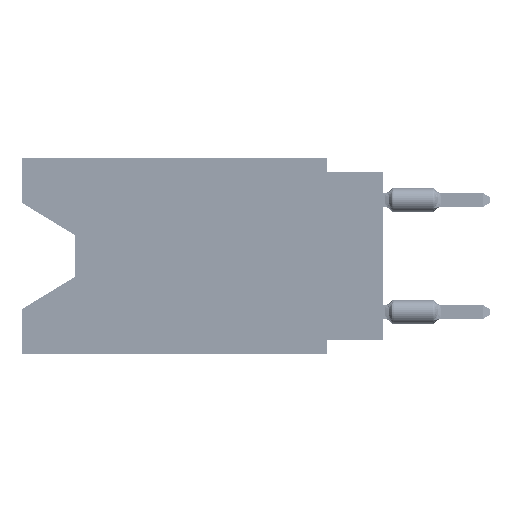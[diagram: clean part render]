
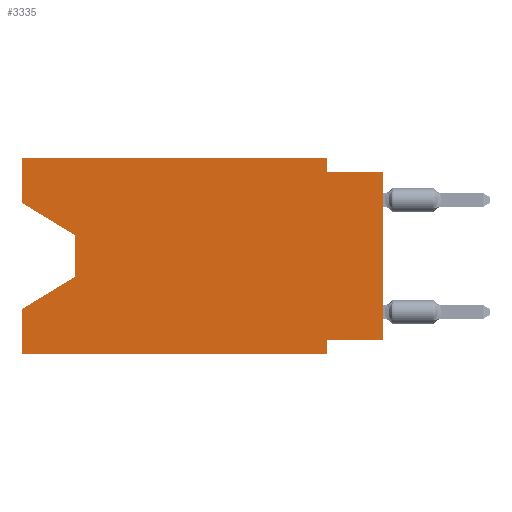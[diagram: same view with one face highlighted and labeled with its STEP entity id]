
A CAD part, left-side view. The second image highlights one B-rep face of the part: STEP entity #3335.
In plain terms, the highlighted planar face has unit normal (-1, 0, 0).
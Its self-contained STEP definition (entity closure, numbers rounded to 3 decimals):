
#1434 = VECTOR ( 'NONE', #78253, 1000. ) ;
#2372 = DIRECTION ( 'NONE',  ( 0., 0., 1. ) ) ;
#2408 = CARTESIAN_POINT ( 'NONE',  ( 0., 2.54, -8.89 ) ) ;
#3335 = ADVANCED_FACE ( 'NONE', ( #8210 ), #54023, .F. ) ;
#4043 = CARTESIAN_POINT ( 'NONE',  ( 0., 2.54, -8.255 ) ) ;
#4222 = CARTESIAN_POINT ( 'NONE',  ( 0., 13.97, -3.505 ) ) ;
#4319 = ORIENTED_EDGE ( 'NONE', *, *, #28063, .T. ) ;
#4534 = CARTESIAN_POINT ( 'NONE',  ( 0., 16.383, 0. ) ) ;
#5040 = VERTEX_POINT ( 'NONE', #15815 ) ;
#5159 = EDGE_CURVE ( 'NONE', #13364, #27211, #65156, .T. ) ;
#6820 = ORIENTED_EDGE ( 'NONE', *, *, #26984, .F. ) ;
#7956 = ORIENTED_EDGE ( 'NONE', *, *, #25380, .F. ) ;
#8210 = FACE_OUTER_BOUND ( 'NONE', #95377, .T. ) ;
#11842 = VECTOR ( 'NONE', #2372, 1000. ) ;
#13364 = VERTEX_POINT ( 'NONE', #4043 ) ;
#14404 = DIRECTION ( 'NONE',  ( 1., 0., 0. ) ) ;
#15815 = CARTESIAN_POINT ( 'NONE',  ( 0., 2.54, 0. ) ) ;
#16827 = LINE ( 'NONE', #69798, #61258 ) ;
#18329 = CARTESIAN_POINT ( 'NONE',  ( 0., 16.383, 0. ) ) ;
#19487 = DIRECTION ( 'NONE',  ( 0., 0., 1. ) ) ;
#21357 = LINE ( 'NONE', #44522, #70945 ) ;
#21946 = LINE ( 'NONE', #36898, #83533 ) ;
#22635 = VERTEX_POINT ( 'NONE', #92030 ) ;
#23181 = ORIENTED_EDGE ( 'NONE', *, *, #52454, .F. ) ;
#24515 = LINE ( 'NONE', #71308, #79455 ) ;
#24968 = LINE ( 'NONE', #56351, #52146 ) ;
#25139 = CARTESIAN_POINT ( 'NONE',  ( 0., 16.383, -2.038 ) ) ;
#25380 = EDGE_CURVE ( 'NONE', #52157, #38865, #67290, .T. ) ;
#26080 = ORIENTED_EDGE ( 'NONE', *, *, #46748, .T. ) ;
#26580 = DIRECTION ( 'NONE',  ( 0., 0., -1. ) ) ;
#26619 = ORIENTED_EDGE ( 'NONE', *, *, #60736, .F. ) ;
#26761 = LINE ( 'NONE', #58156, #28626 ) ;
#26984 = EDGE_CURVE ( 'NONE', #52255, #100583, #41485, .T. ) ;
#27113 = EDGE_CURVE ( 'NONE', #38865, #5040, #21357, .T. ) ;
#27211 = VERTEX_POINT ( 'NONE', #100508 ) ;
#28063 = EDGE_CURVE ( 'NONE', #72103, #22635, #16827, .T. ) ;
#28486 = ORIENTED_EDGE ( 'NONE', *, *, #5159, .F. ) ;
#28626 = VECTOR ( 'NONE', #76590, 1000. ) ;
#29476 = ORIENTED_EDGE ( 'NONE', *, *, #55083, .F. ) ;
#30838 = CARTESIAN_POINT ( 'NONE',  ( 0., 16.383, 0. ) ) ;
#36898 = CARTESIAN_POINT ( 'NONE',  ( 0., 0., -0.635 ) ) ;
#38865 = VERTEX_POINT ( 'NONE', #52210 ) ;
#39980 = DIRECTION ( 'NONE',  ( 0., 0., 1. ) ) ;
#41189 = CARTESIAN_POINT ( 'NONE',  ( 0., 13.97, -5.385 ) ) ;
#41299 = EDGE_CURVE ( 'NONE', #52255, #27211, #43135, .T. ) ;
#41485 = LINE ( 'NONE', #18329, #11842 ) ;
#43135 = LINE ( 'NONE', #56551, #51326 ) ;
#43632 = DIRECTION ( 'NONE',  ( 0., 0., -1. ) ) ;
#44522 = CARTESIAN_POINT ( 'NONE',  ( 0., 16.383, 0. ) ) ;
#44671 = VECTOR ( 'NONE', #19487, 1000. ) ;
#46395 = CARTESIAN_POINT ( 'NONE',  ( 0., 16.383, -2.038 ) ) ;
#46748 = EDGE_CURVE ( 'NONE', #57354, #81608, #59083, .T. ) ;
#46995 = VECTOR ( 'NONE', #26580, 1000. ) ;
#51326 = VECTOR ( 'NONE', #57060, 1000. ) ;
#52146 = VECTOR ( 'NONE', #79989, 1000. ) ;
#52157 = VERTEX_POINT ( 'NONE', #25139 ) ;
#52210 = CARTESIAN_POINT ( 'NONE',  ( 0., 16.383, 0. ) ) ;
#52255 = VERTEX_POINT ( 'NONE', #98099 ) ;
#52454 = EDGE_CURVE ( 'NONE', #72103, #13364, #24515, .T. ) ;
#52747 = DIRECTION ( 'NONE',  ( 0., -1., 0. ) ) ;
#53680 = CARTESIAN_POINT ( 'NONE',  ( 0., 2.54, -0.635 ) ) ;
#54023 = PLANE ( 'NONE',  #91399 ) ;
#55083 = EDGE_CURVE ( 'NONE', #5040, #66073, #26761, .T. ) ;
#55945 = ORIENTED_EDGE ( 'NONE', *, *, #27113, .F. ) ;
#56351 = CARTESIAN_POINT ( 'NONE',  ( 0., 13.97, -5.385 ) ) ;
#56551 = CARTESIAN_POINT ( 'NONE',  ( 0., 16.383, -8.89 ) ) ;
#57060 = DIRECTION ( 'NONE',  ( 0., -1., 0. ) ) ;
#57354 = VERTEX_POINT ( 'NONE', #4222 ) ;
#57996 = EDGE_CURVE ( 'NONE', #81608, #100583, #24968, .T. ) ;
#58156 = CARTESIAN_POINT ( 'NONE',  ( 0., 2.54, 0. ) ) ;
#59083 = LINE ( 'NONE', #90409, #71747 ) ;
#60736 = EDGE_CURVE ( 'NONE', #66073, #22635, #21946, .T. ) ;
#61133 = EDGE_CURVE ( 'NONE', #52157, #57354, #61819, .T. ) ;
#61258 = VECTOR ( 'NONE', #39980, 1000. ) ;
#61819 = LINE ( 'NONE', #46395, #1434 ) ;
#62226 = DIRECTION ( 'NONE',  ( 0., 0., -1. ) ) ;
#65156 = LINE ( 'NONE', #2408, #46995 ) ;
#66073 = VERTEX_POINT ( 'NONE', #53680 ) ;
#67290 = LINE ( 'NONE', #4534, #44671 ) ;
#69798 = CARTESIAN_POINT ( 'NONE',  ( 0., 0., 0. ) ) ;
#70278 = DIRECTION ( 'NONE',  ( 0., -1., 0. ) ) ;
#70945 = VECTOR ( 'NONE', #52747, 1000. ) ;
#71308 = CARTESIAN_POINT ( 'NONE',  ( 0., 0., -8.255 ) ) ;
#71747 = VECTOR ( 'NONE', #43632, 1000. ) ;
#72103 = VERTEX_POINT ( 'NONE', #76086 ) ;
#76086 = CARTESIAN_POINT ( 'NONE',  ( 0., 0., -8.255 ) ) ;
#76590 = DIRECTION ( 'NONE',  ( 0., 0., -1. ) ) ;
#76658 = ORIENTED_EDGE ( 'NONE', *, *, #57996, .T. ) ;
#78253 = DIRECTION ( 'NONE',  ( 0., -0.855, -0.519 ) ) ;
#79455 = VECTOR ( 'NONE', #93938, 1000. ) ;
#79989 = DIRECTION ( 'NONE',  ( 0., 0.855, -0.519 ) ) ;
#81553 = CARTESIAN_POINT ( 'NONE',  ( 0., 16.383, -6.852 ) ) ;
#81608 = VERTEX_POINT ( 'NONE', #41189 ) ;
#82467 = ORIENTED_EDGE ( 'NONE', *, *, #41299, .T. ) ;
#83533 = VECTOR ( 'NONE', #70278, 1000. ) ;
#90409 = CARTESIAN_POINT ( 'NONE',  ( 0., 13.97, -3.505 ) ) ;
#91399 = AXIS2_PLACEMENT_3D ( 'NONE', #30838, #14404, #62226 ) ;
#92030 = CARTESIAN_POINT ( 'NONE',  ( 0., 0., -0.635 ) ) ;
#93938 = DIRECTION ( 'NONE',  ( 0., 1., 0. ) ) ;
#95377 = EDGE_LOOP ( 'NONE', ( #98562, #26080, #76658, #6820, #82467, #28486, #23181, #4319, #26619, #29476, #55945, #7956 ) ) ;
#98099 = CARTESIAN_POINT ( 'NONE',  ( 0., 16.383, -8.89 ) ) ;
#98562 = ORIENTED_EDGE ( 'NONE', *, *, #61133, .T. ) ;
#100508 = CARTESIAN_POINT ( 'NONE',  ( 0., 2.54, -8.89 ) ) ;
#100583 = VERTEX_POINT ( 'NONE', #81553 ) ;
